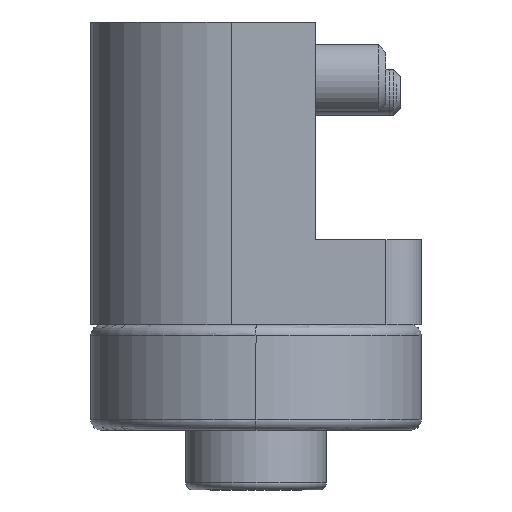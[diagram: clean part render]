
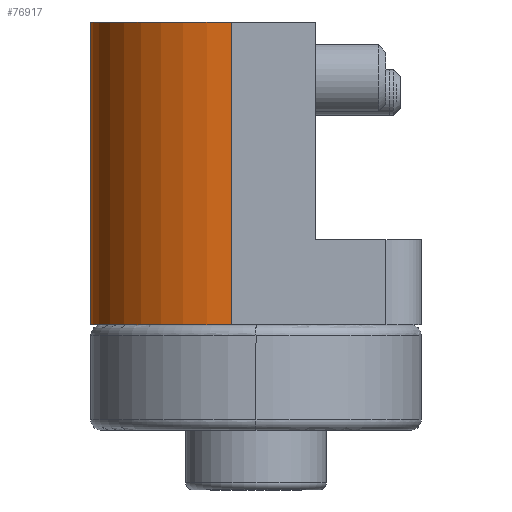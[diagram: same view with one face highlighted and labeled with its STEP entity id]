
A CAD part, left-side view. The second image highlights one B-rep face of the part: STEP entity #76917.
In plain terms, the highlighted cylindrical face has radius 2 mm (diameter 4 mm), a partial arc.
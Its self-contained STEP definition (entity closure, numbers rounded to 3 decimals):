
#2634 = AXIS2_PLACEMENT_3D ( 'NONE', #7654, #34091, #60515 ) ;
#2756 = CARTESIAN_POINT ( 'NONE',  ( -7.5, 0.35, 3.1 ) ) ;
#3687 = ORIENTED_EDGE ( 'NONE', *, *, #65342, .F. ) ;
#7654 = CARTESIAN_POINT ( 'NONE',  ( -5.5, 0.35, 3.1 ) ) ;
#7721 = ORIENTED_EDGE ( 'NONE', *, *, #74490, .T. ) ;
#8338 = CARTESIAN_POINT ( 'NONE',  ( -5.5, 0.35, 3.186 ) ) ;
#9621 = VERTEX_POINT ( 'NONE', #16131 ) ;
#9852 = CARTESIAN_POINT ( 'NONE',  ( -7.5, 0.35, -1.21 ) ) ;
#12008 = DIRECTION ( 'NONE',  ( 0., 1., 0. ) ) ;
#13958 = ORIENTED_EDGE ( 'NONE', *, *, #34087, .F. ) ;
#16131 = CARTESIAN_POINT ( 'NONE',  ( -5.5, 2.35, 3.1 ) ) ;
#18185 = VERTEX_POINT ( 'NONE', #2756 ) ;
#18907 = DIRECTION ( 'NONE',  ( 0., 0., -1. ) ) ;
#22264 = EDGE_LOOP ( 'NONE', ( #77639, #7721, #3687, #13958 ) ) ;
#22845 = LINE ( 'NONE', #49281, #25504 ) ;
#24995 = CARTESIAN_POINT ( 'NONE',  ( -5.5, 0.35, -1.21 ) ) ;
#25504 = VECTOR ( 'NONE', #75710, 1000. ) ;
#33059 = AXIS2_PLACEMENT_3D ( 'NONE', #24995, #71374, #12008 ) ;
#34087 = EDGE_CURVE ( 'NONE', #9621, #18185, #40029, .T. ) ;
#34091 = DIRECTION ( 'NONE',  ( 0., 0., 1. ) ) ;
#34789 = DIRECTION ( 'NONE',  ( 0., 0., -1. ) ) ;
#40029 = CIRCLE ( 'NONE', #2634, 2. ) ;
#41293 = FACE_OUTER_BOUND ( 'NONE', #22264, .T. ) ;
#49281 = CARTESIAN_POINT ( 'NONE',  ( -5.5, 2.35, -1.21 ) ) ;
#51818 = LINE ( 'NONE', #78262, #72285 ) ;
#53769 = VERTEX_POINT ( 'NONE', #82602 ) ;
#55461 = AXIS2_PLACEMENT_3D ( 'NONE', #8338, #34789, #61213 ) ;
#60515 = DIRECTION ( 'NONE',  ( 0., 1., 0. ) ) ;
#61213 = DIRECTION ( 'NONE',  ( -1., 0., 0. ) ) ;
#65342 = EDGE_CURVE ( 'NONE', #18185, #84801, #51818, .T. ) ;
#67633 = EDGE_CURVE ( 'NONE', #53769, #9621, #22845, .T. ) ;
#67713 = CYLINDRICAL_SURFACE ( 'NONE', #55461, 2. ) ;
#70437 = CIRCLE ( 'NONE', #33059, 2. ) ;
#71374 = DIRECTION ( 'NONE',  ( 0., 0., 1. ) ) ;
#72285 = VECTOR ( 'NONE', #18907, 1000. ) ;
#74490 = EDGE_CURVE ( 'NONE', #53769, #84801, #70437, .T. ) ;
#75710 = DIRECTION ( 'NONE',  ( 0., 0., 1. ) ) ;
#76917 = ADVANCED_FACE ( 'NONE', ( #41293 ), #67713, .T. ) ;
#77639 = ORIENTED_EDGE ( 'NONE', *, *, #67633, .F. ) ;
#78262 = CARTESIAN_POINT ( 'NONE',  ( -7.5, 0.35, 3.1 ) ) ;
#82602 = CARTESIAN_POINT ( 'NONE',  ( -5.5, 2.35, -1.21 ) ) ;
#84801 = VERTEX_POINT ( 'NONE', #9852 ) ;
